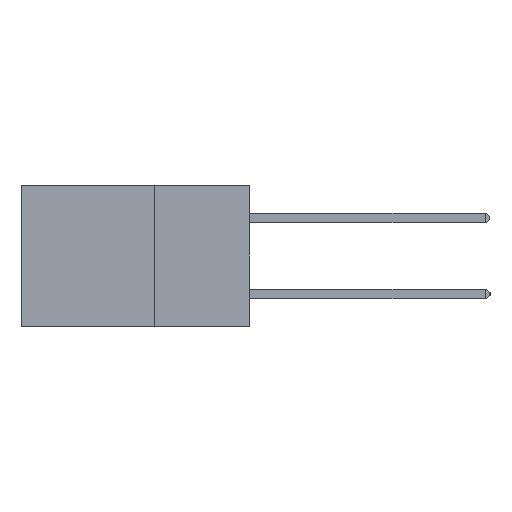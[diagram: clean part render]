
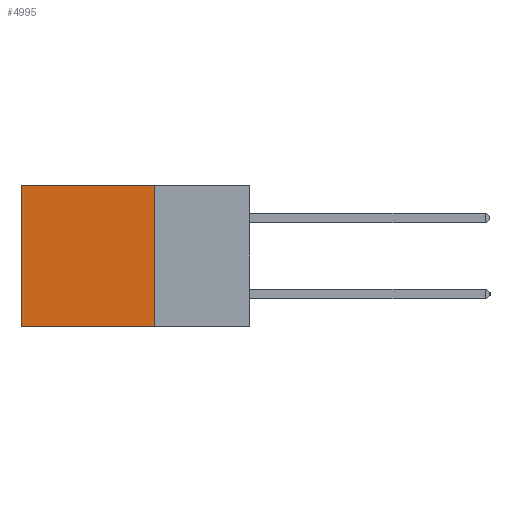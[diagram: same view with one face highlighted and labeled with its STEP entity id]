
A CAD part, left-side view. The second image highlights one B-rep face of the part: STEP entity #4995.
In plain terms, the highlighted planar face has unit normal (-1, 0, 0).
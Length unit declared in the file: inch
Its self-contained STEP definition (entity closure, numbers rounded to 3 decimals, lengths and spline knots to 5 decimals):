
#211 = VECTOR ( 'NONE', #5304, 39.37008 ) ;
#1231 = EDGE_CURVE ( 'NONE', #14283, #22568, #4961, .T. ) ;
#1552 = ORIENTED_EDGE ( 'NONE', *, *, #16450, .T. ) ;
#2122 = LINE ( 'NONE', #17593, #20548 ) ;
#3155 = AXIS2_PLACEMENT_3D ( 'NONE', #22584, #4910, #17383 ) ;
#3636 = CARTESIAN_POINT ( 'NONE',  ( 0.2875, 0.6, 0. ) ) ;
#3665 = CARTESIAN_POINT ( 'NONE',  ( 0.2875, 0.25, -0.37 ) ) ;
#4910 = DIRECTION ( 'NONE',  ( 1., 0., 0. ) ) ;
#4961 = LINE ( 'NONE', #11464, #18620 ) ;
#4995 = ADVANCED_FACE ( 'NONE', ( #17940 ), #15625, .F. ) ;
#5152 = EDGE_CURVE ( 'NONE', #6466, #17265, #14665, .T. ) ;
#5304 = DIRECTION ( 'NONE',  ( 0., 0., -1. ) ) ;
#6466 = VERTEX_POINT ( 'NONE', #13839 ) ;
#7200 = CARTESIAN_POINT ( 'NONE',  ( 0.2875, 0.6, -0.37 ) ) ;
#9465 = EDGE_CURVE ( 'NONE', #17265, #22568, #10588, .T. ) ;
#10031 = VECTOR ( 'NONE', #16913, 39.37008 ) ;
#10227 = ORIENTED_EDGE ( 'NONE', *, *, #9465, .F. ) ;
#10588 = LINE ( 'NONE', #15164, #10031 ) ;
#11464 = CARTESIAN_POINT ( 'NONE',  ( 0.2875, 0.6, 0. ) ) ;
#12826 = ORIENTED_EDGE ( 'NONE', *, *, #1231, .T. ) ;
#13258 = DIRECTION ( 'NONE',  ( 0., 0., -1. ) ) ;
#13839 = CARTESIAN_POINT ( 'NONE',  ( 0.2875, 0.25, 0. ) ) ;
#14267 = CARTESIAN_POINT ( 'NONE',  ( 0.2875, 0.25, 0. ) ) ;
#14283 = VERTEX_POINT ( 'NONE', #3636 ) ;
#14665 = LINE ( 'NONE', #14267, #211 ) ;
#15164 = CARTESIAN_POINT ( 'NONE',  ( 0.2875, 0.25, -0.37 ) ) ;
#15448 = EDGE_LOOP ( 'NONE', ( #12826, #10227, #19650, #1552 ) ) ;
#15625 = PLANE ( 'NONE',  #3155 ) ;
#16450 = EDGE_CURVE ( 'NONE', #6466, #14283, #2122, .T. ) ;
#16913 = DIRECTION ( 'NONE',  ( 0., 1., 0. ) ) ;
#17265 = VERTEX_POINT ( 'NONE', #3665 ) ;
#17383 = DIRECTION ( 'NONE',  ( 0., 0., -1. ) ) ;
#17593 = CARTESIAN_POINT ( 'NONE',  ( 0.2875, 0.25, 0. ) ) ;
#17940 = FACE_OUTER_BOUND ( 'NONE', #15448, .T. ) ;
#18620 = VECTOR ( 'NONE', #13258, 39.37008 ) ;
#19650 = ORIENTED_EDGE ( 'NONE', *, *, #5152, .F. ) ;
#20548 = VECTOR ( 'NONE', #21107, 39.37008 ) ;
#21107 = DIRECTION ( 'NONE',  ( 0., 1., 0. ) ) ;
#22568 = VERTEX_POINT ( 'NONE', #7200 ) ;
#22584 = CARTESIAN_POINT ( 'NONE',  ( 0.2875, 0.25, 0. ) ) ;
